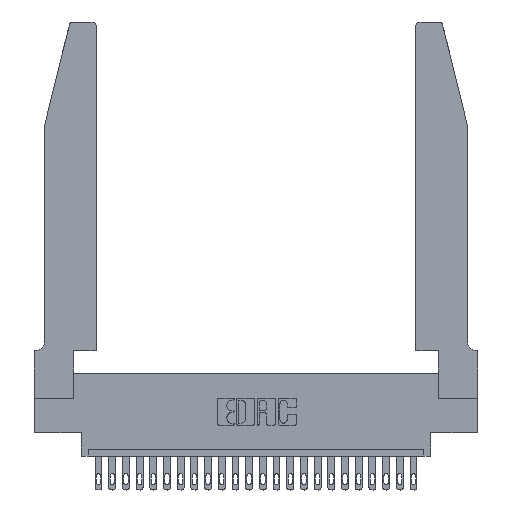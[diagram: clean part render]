
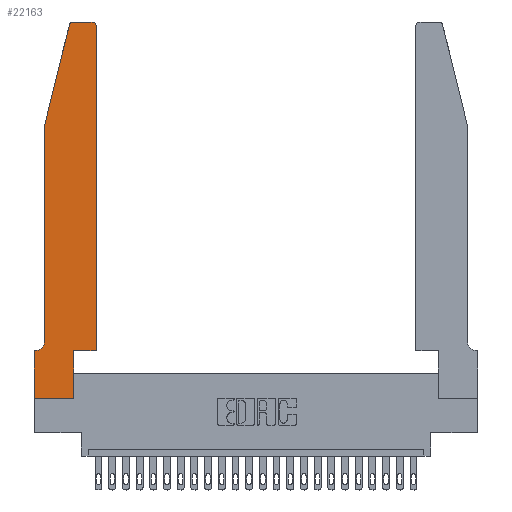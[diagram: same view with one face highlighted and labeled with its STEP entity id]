
A CAD part, top view. The second image highlights one B-rep face of the part: STEP entity #22163.
In plain terms, the highlighted planar face has unit normal (0, 0, 1).
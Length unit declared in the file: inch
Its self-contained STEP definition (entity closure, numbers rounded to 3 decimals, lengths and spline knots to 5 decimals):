
#11 = PLANE ( 'NONE',  #10897 ) ;
#178 = CARTESIAN_POINT ( 'NONE',  ( 0.0055, 0.35, 0.37 ) ) ;
#373 = CARTESIAN_POINT ( 'NONE',  ( 0., 0., 0.37 ) ) ;
#464 = VECTOR ( 'NONE', #12711, 39.37008 ) ;
#791 = CARTESIAN_POINT ( 'NONE',  ( 0.2605, 2.75, 0.37 ) ) ;
#878 = EDGE_CURVE ( 'NONE', #15485, #8023, #21078, .T. ) ;
#938 = AXIS2_PLACEMENT_3D ( 'NONE', #15064, #16910, #24601 ) ;
#1100 = LINE ( 'NONE', #24423, #464 ) ;
#1166 = VERTEX_POINT ( 'NONE', #178 ) ;
#1183 = LINE ( 'NONE', #4513, #21349 ) ;
#1480 = ORIENTED_EDGE ( 'NONE', *, *, #24787, .T. ) ;
#1685 = CARTESIAN_POINT ( 'NONE',  ( 0.0055, 0.42, 0.37 ) ) ;
#1734 = VERTEX_POINT ( 'NONE', #18245 ) ;
#2385 = VERTEX_POINT ( 'NONE', #21337 ) ;
#2581 = CARTESIAN_POINT ( 'NONE',  ( 0.0755, 2., 0.37 ) ) ;
#3166 = VERTEX_POINT ( 'NONE', #6941 ) ;
#3364 = CARTESIAN_POINT ( 'NONE',  ( 0.4505, 0.35, 0.37 ) ) ;
#3406 = DIRECTION ( 'NONE',  ( 0., 1., 0. ) ) ;
#3920 = EDGE_CURVE ( 'NONE', #21063, #2385, #7020, .T. ) ;
#4513 = CARTESIAN_POINT ( 'NONE',  ( 0., 0., 0.37 ) ) ;
#4633 = LINE ( 'NONE', #3364, #23577 ) ;
#4775 = EDGE_CURVE ( 'NONE', #3166, #21063, #1183, .T. ) ;
#5026 = ORIENTED_EDGE ( 'NONE', *, *, #14817, .T. ) ;
#5435 = EDGE_CURVE ( 'NONE', #25090, #20381, #13358, .T. ) ;
#5439 = DIRECTION ( 'NONE',  ( 0., 0., -1. ) ) ;
#5722 = LINE ( 'NONE', #791, #17343 ) ;
#6049 = CARTESIAN_POINT ( 'NONE',  ( 0.4505, 0.35, 0.37 ) ) ;
#6067 = VECTOR ( 'NONE', #21030, 39.37008 ) ;
#6941 = CARTESIAN_POINT ( 'NONE',  ( 0., 0.35, 0.37 ) ) ;
#7020 = LINE ( 'NONE', #20681, #6067 ) ;
#7126 = CARTESIAN_POINT ( 'NONE',  ( 0.0755, 2., 0.37 ) ) ;
#7682 = ORIENTED_EDGE ( 'NONE', *, *, #878, .T. ) ;
#8023 = VERTEX_POINT ( 'NONE', #6049 ) ;
#8555 = DIRECTION ( 'NONE',  ( -1., 0., 0. ) ) ;
#9683 = ORIENTED_EDGE ( 'NONE', *, *, #3920, .T. ) ;
#9740 = CARTESIAN_POINT ( 'NONE',  ( 0.284, 2.72, 0.37 ) ) ;
#10087 = VERTEX_POINT ( 'NONE', #14081 ) ;
#10118 = VERTEX_POINT ( 'NONE', #24597 ) ;
#10462 = ORIENTED_EDGE ( 'NONE', *, *, #21423, .T. ) ;
#10897 = AXIS2_PLACEMENT_3D ( 'NONE', #23323, #11594, #17515 ) ;
#11366 = ORIENTED_EDGE ( 'NONE', *, *, #5435, .T. ) ;
#11430 = CARTESIAN_POINT ( 'NONE',  ( 0.2865, 0.35, 0.37 ) ) ;
#11594 = DIRECTION ( 'NONE',  ( 0., 0., 1. ) ) ;
#12711 = DIRECTION ( 'NONE',  ( 0., -1., 0. ) ) ;
#12823 = CIRCLE ( 'NONE', #938, 0.03 ) ;
#13131 = VECTOR ( 'NONE', #13572, 39.37008 ) ;
#13358 = LINE ( 'NONE', #7126, #24351 ) ;
#13572 = DIRECTION ( 'NONE',  ( 1., 0., 0. ) ) ;
#13723 = CARTESIAN_POINT ( 'NONE',  ( 0.4505, 0.35, 0.37 ) ) ;
#14081 = CARTESIAN_POINT ( 'NONE',  ( 0.0755, 0.42, 0.37 ) ) ;
#14209 = VECTOR ( 'NONE', #3406, 39.37008 ) ;
#14266 = CARTESIAN_POINT ( 'NONE',  ( 0.4205, 2.75, 0.37 ) ) ;
#14358 = CARTESIAN_POINT ( 'NONE',  ( 0.2865, 0.35, 0.37 ) ) ;
#14456 = ORIENTED_EDGE ( 'NONE', *, *, #20527, .T. ) ;
#14558 = CIRCLE ( 'NONE', #21187, 0.03 ) ;
#14629 = EDGE_CURVE ( 'NONE', #20381, #10087, #1100, .T. ) ;
#14673 = ORIENTED_EDGE ( 'NONE', *, *, #14629, .T. ) ;
#14817 = EDGE_CURVE ( 'NONE', #2385, #15485, #23991, .T. ) ;
#15064 = CARTESIAN_POINT ( 'NONE',  ( 0.4205, 2.72, 0.37 ) ) ;
#15191 = ORIENTED_EDGE ( 'NONE', *, *, #20797, .T. ) ;
#15485 = VERTEX_POINT ( 'NONE', #14358 ) ;
#15683 = ORIENTED_EDGE ( 'NONE', *, *, #22389, .T. ) ;
#15769 = CARTESIAN_POINT ( 'NONE',  ( 0.25487, 2.72718, 0.37 ) ) ;
#15798 = AXIS2_PLACEMENT_3D ( 'NONE', #1685, #5439, #19125 ) ;
#15925 = FACE_OUTER_BOUND ( 'NONE', #21123, .T. ) ;
#16910 = DIRECTION ( 'NONE',  ( 0., 0., 1. ) ) ;
#16957 = DIRECTION ( 'NONE',  ( -0.239, -0.971, 0. ) ) ;
#17040 = EDGE_CURVE ( 'NONE', #1166, #3166, #21760, .T. ) ;
#17049 = DIRECTION ( 'NONE',  ( 0., 1., 0. ) ) ;
#17217 = DIRECTION ( 'NONE',  ( 1., 0., 0. ) ) ;
#17343 = VECTOR ( 'NONE', #18561, 39.37008 ) ;
#17515 = DIRECTION ( 'NONE',  ( 1., 0., 0. ) ) ;
#18110 = VECTOR ( 'NONE', #8555, 39.37008 ) ;
#18245 = CARTESIAN_POINT ( 'NONE',  ( 0.284, 2.75, 0.37 ) ) ;
#18561 = DIRECTION ( 'NONE',  ( -1., 0., 0. ) ) ;
#19125 = DIRECTION ( 'NONE',  ( -1., 0., 0. ) ) ;
#19396 = VERTEX_POINT ( 'NONE', #14266 ) ;
#19543 = ORIENTED_EDGE ( 'NONE', *, *, #17040, .T. ) ;
#20381 = VERTEX_POINT ( 'NONE', #2581 ) ;
#20527 = EDGE_CURVE ( 'NONE', #19396, #1734, #5722, .T. ) ;
#20681 = CARTESIAN_POINT ( 'NONE',  ( 0., 0., 0.37 ) ) ;
#20797 = EDGE_CURVE ( 'NONE', #1734, #25090, #14558, .T. ) ;
#21030 = DIRECTION ( 'NONE',  ( 1., 0., 0. ) ) ;
#21063 = VERTEX_POINT ( 'NONE', #373 ) ;
#21078 = LINE ( 'NONE', #13723, #13131 ) ;
#21123 = EDGE_LOOP ( 'NONE', ( #14456, #15191, #11366, #14673, #15683, #19543, #23102, #9683, #5026, #7682, #10462, #1480 ) ) ;
#21187 = AXIS2_PLACEMENT_3D ( 'NONE', #9740, #23176, #17217 ) ;
#21337 = CARTESIAN_POINT ( 'NONE',  ( 0.2865, 0., 0.37 ) ) ;
#21349 = VECTOR ( 'NONE', #21839, 39.37008 ) ;
#21423 = EDGE_CURVE ( 'NONE', #8023, #10118, #4633, .T. ) ;
#21760 = LINE ( 'NONE', #22102, #18110 ) ;
#21839 = DIRECTION ( 'NONE',  ( 0., -1., 0. ) ) ;
#22102 = CARTESIAN_POINT ( 'NONE',  ( 0.0755, 0.35, 0.37 ) ) ;
#22163 = ADVANCED_FACE ( 'NONE', ( #15925 ), #11, .T. ) ;
#22389 = EDGE_CURVE ( 'NONE', #10087, #1166, #23552, .T. ) ;
#23102 = ORIENTED_EDGE ( 'NONE', *, *, #4775, .T. ) ;
#23176 = DIRECTION ( 'NONE',  ( 0., 0., 1. ) ) ;
#23323 = CARTESIAN_POINT ( 'NONE',  ( 0., 0.35, 0.37 ) ) ;
#23552 = CIRCLE ( 'NONE', #15798, 0.07 ) ;
#23577 = VECTOR ( 'NONE', #17049, 39.37008 ) ;
#23991 = LINE ( 'NONE', #11430, #14209 ) ;
#24351 = VECTOR ( 'NONE', #16957, 39.37008 ) ;
#24423 = CARTESIAN_POINT ( 'NONE',  ( 0.0755, 2., 0.37 ) ) ;
#24597 = CARTESIAN_POINT ( 'NONE',  ( 0.4505, 2.72, 0.37 ) ) ;
#24601 = DIRECTION ( 'NONE',  ( 1., 0., 0. ) ) ;
#24787 = EDGE_CURVE ( 'NONE', #10118, #19396, #12823, .T. ) ;
#25090 = VERTEX_POINT ( 'NONE', #15769 ) ;
